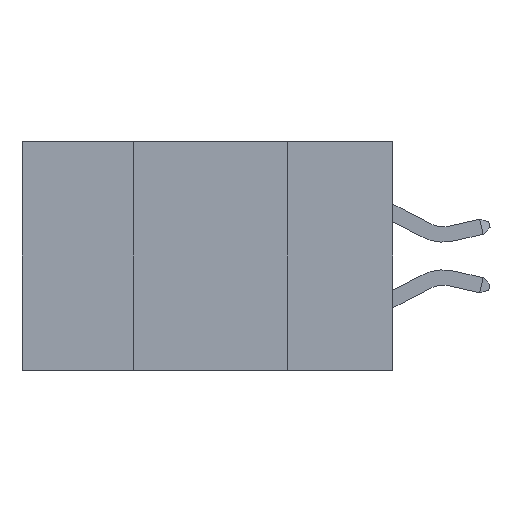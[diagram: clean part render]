
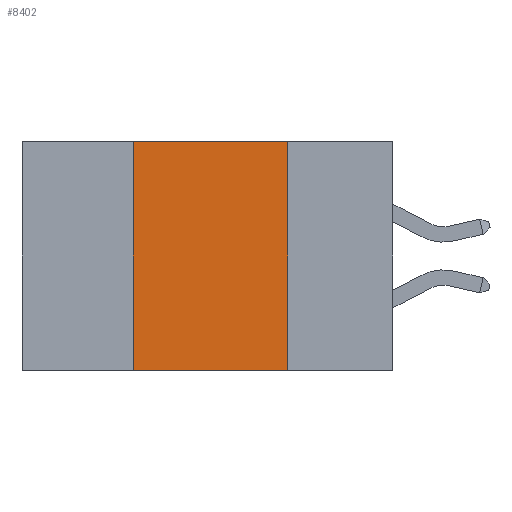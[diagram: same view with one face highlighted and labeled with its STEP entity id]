
A CAD part, left-side view. The second image highlights one B-rep face of the part: STEP entity #8402.
In plain terms, the highlighted planar face has unit normal (-1, 0, 0).
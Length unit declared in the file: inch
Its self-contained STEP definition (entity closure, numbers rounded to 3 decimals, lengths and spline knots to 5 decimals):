
#326 = DIRECTION ( 'NONE',  ( 0., -1., 0. ) ) ;
#1436 = VECTOR ( 'NONE', #3694, 39.37008 ) ;
#1586 = VERTEX_POINT ( 'NONE', #8425 ) ;
#1870 = PLANE ( 'NONE',  #10149 ) ;
#2262 = CARTESIAN_POINT ( 'NONE',  ( 0., 0.42, -0.37 ) ) ;
#2379 = DIRECTION ( 'NONE',  ( 0., 0., -1. ) ) ;
#2738 = LINE ( 'NONE', #10804, #1436 ) ;
#3039 = CARTESIAN_POINT ( 'NONE',  ( 0., 0.17, -0.37 ) ) ;
#3280 = CARTESIAN_POINT ( 'NONE',  ( 0., 0.6, 0. ) ) ;
#3692 = EDGE_CURVE ( 'NONE', #17635, #15603, #15809, .T. ) ;
#3694 = DIRECTION ( 'NONE',  ( 0., 0., 1. ) ) ;
#3841 = EDGE_CURVE ( 'NONE', #1586, #16527, #9574, .T. ) ;
#4038 = EDGE_CURVE ( 'NONE', #16527, #15603, #4311, .T. ) ;
#4064 = ORIENTED_EDGE ( 'NONE', *, *, #4038, .F. ) ;
#4074 = EDGE_LOOP ( 'NONE', ( #4064, #11576, #4169, #15518 ) ) ;
#4169 = ORIENTED_EDGE ( 'NONE', *, *, #5198, .F. ) ;
#4311 = LINE ( 'NONE', #10983, #16237 ) ;
#4552 = CARTESIAN_POINT ( 'NONE',  ( 0., 0.6, -0.37 ) ) ;
#5198 = EDGE_CURVE ( 'NONE', #17635, #1586, #2738, .T. ) ;
#6452 = CARTESIAN_POINT ( 'NONE',  ( 0., 0.6, 0. ) ) ;
#8144 = FACE_OUTER_BOUND ( 'NONE', #4074, .T. ) ;
#8402 = ADVANCED_FACE ( 'NONE', ( #8144 ), #1870, .F. ) ;
#8425 = CARTESIAN_POINT ( 'NONE',  ( 0., 0.42, 0. ) ) ;
#9217 = CARTESIAN_POINT ( 'NONE',  ( 0., 0.17, 0. ) ) ;
#9574 = LINE ( 'NONE', #6452, #14233 ) ;
#10149 = AXIS2_PLACEMENT_3D ( 'NONE', #3280, #15744, #13132 ) ;
#10250 = VECTOR ( 'NONE', #326, 39.37008 ) ;
#10804 = CARTESIAN_POINT ( 'NONE',  ( 0., 0.42, 0. ) ) ;
#10983 = CARTESIAN_POINT ( 'NONE',  ( 0., 0.17, 0. ) ) ;
#11576 = ORIENTED_EDGE ( 'NONE', *, *, #3841, .F. ) ;
#13132 = DIRECTION ( 'NONE',  ( 0., 0., -1. ) ) ;
#14233 = VECTOR ( 'NONE', #16084, 39.37008 ) ;
#15518 = ORIENTED_EDGE ( 'NONE', *, *, #3692, .T. ) ;
#15603 = VERTEX_POINT ( 'NONE', #3039 ) ;
#15744 = DIRECTION ( 'NONE',  ( 1., 0., 0. ) ) ;
#15809 = LINE ( 'NONE', #4552, #10250 ) ;
#16084 = DIRECTION ( 'NONE',  ( 0., -1., 0. ) ) ;
#16237 = VECTOR ( 'NONE', #2379, 39.37008 ) ;
#16527 = VERTEX_POINT ( 'NONE', #9217 ) ;
#17635 = VERTEX_POINT ( 'NONE', #2262 ) ;
